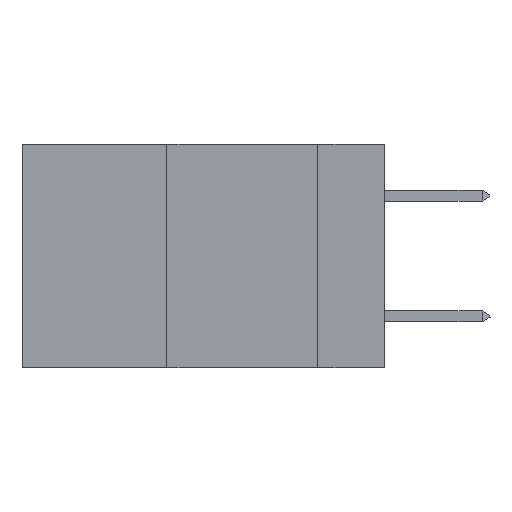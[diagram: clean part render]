
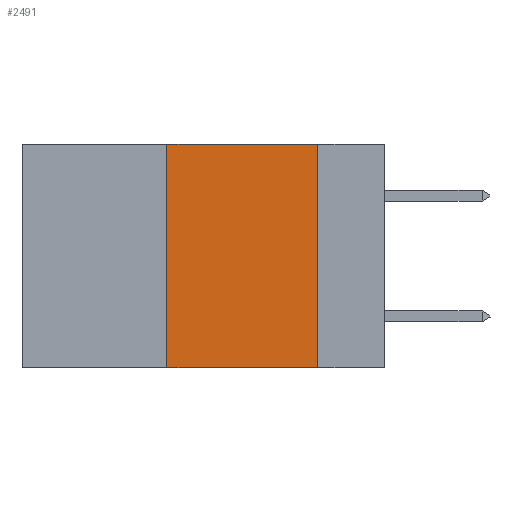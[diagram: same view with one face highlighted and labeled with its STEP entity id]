
A CAD part, left-side view. The second image highlights one B-rep face of the part: STEP entity #2491.
In plain terms, the highlighted planar face has unit normal (-1, 0, 0).
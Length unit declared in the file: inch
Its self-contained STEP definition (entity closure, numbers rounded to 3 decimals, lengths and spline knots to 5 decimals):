
#584 = CARTESIAN_POINT ( 'NONE',  ( 0., 0.36, 0. ) ) ;
#630 = LINE ( 'NONE', #1166, #6502 ) ;
#1166 = CARTESIAN_POINT ( 'NONE',  ( 0., 0.6, -0.37 ) ) ;
#1204 = DIRECTION ( 'NONE',  ( 0., -1., 0. ) ) ;
#1404 = VERTEX_POINT ( 'NONE', #5532 ) ;
#1540 = CARTESIAN_POINT ( 'NONE',  ( 0., 0.6, 0. ) ) ;
#1595 = DIRECTION ( 'NONE',  ( 1., 0., 0. ) ) ;
#1629 = CARTESIAN_POINT ( 'NONE',  ( 0., 0.6, 0. ) ) ;
#2262 = CARTESIAN_POINT ( 'NONE',  ( 0., 0.36, -0.37 ) ) ;
#2304 = ORIENTED_EDGE ( 'NONE', *, *, #2935, .F. ) ;
#2491 = ADVANCED_FACE ( 'NONE', ( #8101 ), #8038, .F. ) ;
#2935 = EDGE_CURVE ( 'NONE', #2988, #5510, #5001, .T. ) ;
#2988 = VERTEX_POINT ( 'NONE', #2262 ) ;
#3019 = DIRECTION ( 'NONE',  ( 0., -1., 0. ) ) ;
#3575 = EDGE_CURVE ( 'NONE', #5510, #1404, #8877, .T. ) ;
#3993 = ORIENTED_EDGE ( 'NONE', *, *, #3575, .F. ) ;
#4419 = EDGE_CURVE ( 'NONE', #2988, #6576, #630, .T. ) ;
#4583 = LINE ( 'NONE', #7823, #7593 ) ;
#5001 = LINE ( 'NONE', #7198, #7669 ) ;
#5182 = ORIENTED_EDGE ( 'NONE', *, *, #6765, .F. ) ;
#5510 = VERTEX_POINT ( 'NONE', #584 ) ;
#5532 = CARTESIAN_POINT ( 'NONE',  ( 0., 0.11, 0. ) ) ;
#5666 = ORIENTED_EDGE ( 'NONE', *, *, #4419, .T. ) ;
#6109 = AXIS2_PLACEMENT_3D ( 'NONE', #1629, #1595, #7302 ) ;
#6156 = EDGE_LOOP ( 'NONE', ( #5182, #3993, #2304, #5666 ) ) ;
#6502 = VECTOR ( 'NONE', #1204, 39.37008 ) ;
#6576 = VERTEX_POINT ( 'NONE', #6783 ) ;
#6765 = EDGE_CURVE ( 'NONE', #1404, #6576, #4583, .T. ) ;
#6783 = CARTESIAN_POINT ( 'NONE',  ( 0., 0.11, -0.37 ) ) ;
#6991 = VECTOR ( 'NONE', #3019, 39.37008 ) ;
#7198 = CARTESIAN_POINT ( 'NONE',  ( 0., 0.36, 0. ) ) ;
#7302 = DIRECTION ( 'NONE',  ( 0., 0., -1. ) ) ;
#7593 = VECTOR ( 'NONE', #8514, 39.37008 ) ;
#7669 = VECTOR ( 'NONE', #7841, 39.37008 ) ;
#7823 = CARTESIAN_POINT ( 'NONE',  ( 0., 0.11, 0. ) ) ;
#7841 = DIRECTION ( 'NONE',  ( 0., 0., 1. ) ) ;
#8038 = PLANE ( 'NONE',  #6109 ) ;
#8101 = FACE_OUTER_BOUND ( 'NONE', #6156, .T. ) ;
#8514 = DIRECTION ( 'NONE',  ( 0., 0., -1. ) ) ;
#8877 = LINE ( 'NONE', #1540, #6991 ) ;
